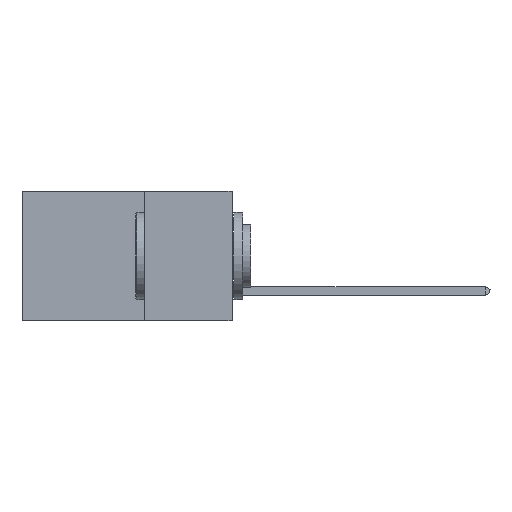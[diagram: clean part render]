
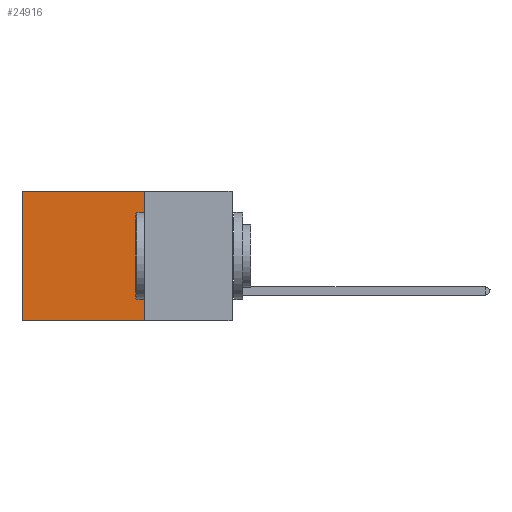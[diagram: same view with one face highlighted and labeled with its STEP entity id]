
A CAD part, left-side view. The second image highlights one B-rep face of the part: STEP entity #24916.
In plain terms, the highlighted planar face has unit normal (-1, 0, 0).
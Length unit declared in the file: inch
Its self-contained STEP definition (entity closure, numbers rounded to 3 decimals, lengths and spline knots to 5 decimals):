
#51 = CARTESIAN_POINT ( 'NONE',  ( 0.2875, 0.25, 0. ) ) ;
#219 = VECTOR ( 'NONE', #18515, 39.37008 ) ;
#398 = VECTOR ( 'NONE', #9132, 39.37008 ) ;
#471 = AXIS2_PLACEMENT_3D ( 'NONE', #51, #21627, #2107 ) ;
#1453 = LINE ( 'NONE', #14466, #219 ) ;
#2107 = DIRECTION ( 'NONE',  ( 0., 0., -1. ) ) ;
#3689 = LINE ( 'NONE', #11055, #17395 ) ;
#3703 = EDGE_CURVE ( 'NONE', #11051, #4375, #3689, .T. ) ;
#4375 = VERTEX_POINT ( 'NONE', #22838 ) ;
#5547 = ORIENTED_EDGE ( 'NONE', *, *, #24733, .F. ) ;
#7700 = ORIENTED_EDGE ( 'NONE', *, *, #3703, .T. ) ;
#7878 = VERTEX_POINT ( 'NONE', #12493 ) ;
#8346 = CARTESIAN_POINT ( 'NONE',  ( 0.2875, 0.6, -0.37 ) ) ;
#9132 = DIRECTION ( 'NONE',  ( 0., 1., 0. ) ) ;
#11051 = VERTEX_POINT ( 'NONE', #25136 ) ;
#11055 = CARTESIAN_POINT ( 'NONE',  ( 0.2875, 0.25, 0. ) ) ;
#12493 = CARTESIAN_POINT ( 'NONE',  ( 0.2875, 0.25, -0.37 ) ) ;
#13496 = EDGE_CURVE ( 'NONE', #4375, #24573, #25058, .T. ) ;
#14466 = CARTESIAN_POINT ( 'NONE',  ( 0.2875, 0.25, 0. ) ) ;
#15013 = DIRECTION ( 'NONE',  ( 0., 1., 0. ) ) ;
#15066 = EDGE_CURVE ( 'NONE', #11051, #7878, #1453, .T. ) ;
#15938 = LINE ( 'NONE', #16988, #398 ) ;
#16846 = FACE_OUTER_BOUND ( 'NONE', #17002, .T. ) ;
#16988 = CARTESIAN_POINT ( 'NONE',  ( 0.2875, 0.25, -0.37 ) ) ;
#17002 = EDGE_LOOP ( 'NONE', ( #19331, #5547, #23684, #7700 ) ) ;
#17395 = VECTOR ( 'NONE', #15013, 39.37008 ) ;
#18515 = DIRECTION ( 'NONE',  ( 0., 0., -1. ) ) ;
#19331 = ORIENTED_EDGE ( 'NONE', *, *, #13496, .T. ) ;
#19616 = CARTESIAN_POINT ( 'NONE',  ( 0.2875, 0.6, 0. ) ) ;
#21627 = DIRECTION ( 'NONE',  ( 1., 0., 0. ) ) ;
#22838 = CARTESIAN_POINT ( 'NONE',  ( 0.2875, 0.6, 0. ) ) ;
#23193 = VECTOR ( 'NONE', #24720, 39.37008 ) ;
#23600 = PLANE ( 'NONE',  #471 ) ;
#23684 = ORIENTED_EDGE ( 'NONE', *, *, #15066, .F. ) ;
#24573 = VERTEX_POINT ( 'NONE', #8346 ) ;
#24720 = DIRECTION ( 'NONE',  ( 0., 0., -1. ) ) ;
#24733 = EDGE_CURVE ( 'NONE', #7878, #24573, #15938, .T. ) ;
#24916 = ADVANCED_FACE ( 'NONE', ( #16846 ), #23600, .F. ) ;
#25058 = LINE ( 'NONE', #19616, #23193 ) ;
#25136 = CARTESIAN_POINT ( 'NONE',  ( 0.2875, 0.25, 0. ) ) ;
